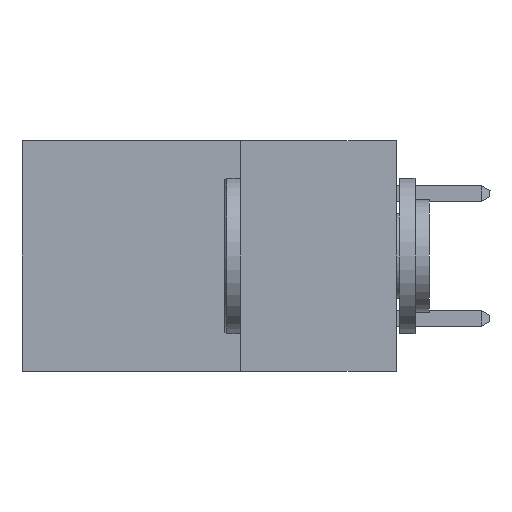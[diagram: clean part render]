
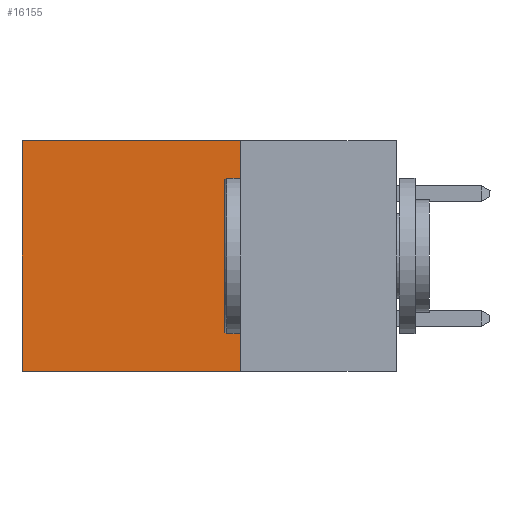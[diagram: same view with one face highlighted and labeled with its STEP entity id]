
A CAD part, left-side view. The second image highlights one B-rep face of the part: STEP entity #16155.
In plain terms, the highlighted planar face has unit normal (-1, 0, 0).
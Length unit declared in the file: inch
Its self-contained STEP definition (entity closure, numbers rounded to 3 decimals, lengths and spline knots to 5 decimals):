
#15 = LINE ( 'NONE', #16534, #13486 ) ;
#3151 = ORIENTED_EDGE ( 'NONE', *, *, #14069, .T. ) ;
#3170 = VECTOR ( 'NONE', #11652, 39.37008 ) ;
#3316 = EDGE_CURVE ( 'NONE', #9972, #3493, #14128, .T. ) ;
#3342 = EDGE_CURVE ( 'NONE', #8411, #16577, #3589, .T. ) ;
#3493 = VERTEX_POINT ( 'NONE', #13466 ) ;
#3589 = LINE ( 'NONE', #11911, #3170 ) ;
#3911 = CARTESIAN_POINT ( 'NONE',  ( 0.298, 0.25, 0. ) ) ;
#5063 = LINE ( 'NONE', #16751, #15480 ) ;
#5919 = ORIENTED_EDGE ( 'NONE', *, *, #3316, .T. ) ;
#6344 = ORIENTED_EDGE ( 'NONE', *, *, #8109, .F. ) ;
#6583 = PLANE ( 'NONE',  #7246 ) ;
#6640 = DIRECTION ( 'NONE',  ( 0., 0., -1. ) ) ;
#7246 = AXIS2_PLACEMENT_3D ( 'NONE', #3911, #14449, #6640 ) ;
#7383 = CARTESIAN_POINT ( 'NONE',  ( 0.298, 0.6, 0. ) ) ;
#7765 = DIRECTION ( 'NONE',  ( 0., 1., 0. ) ) ;
#8109 = EDGE_CURVE ( 'NONE', #16577, #3493, #5063, .T. ) ;
#8411 = VERTEX_POINT ( 'NONE', #10928 ) ;
#8626 = CARTESIAN_POINT ( 'NONE',  ( 0.298, 0.25, -0.37 ) ) ;
#9972 = VERTEX_POINT ( 'NONE', #7383 ) ;
#10173 = DIRECTION ( 'NONE',  ( 0., 1., 0. ) ) ;
#10680 = VECTOR ( 'NONE', #16764, 39.37008 ) ;
#10928 = CARTESIAN_POINT ( 'NONE',  ( 0.298, 0.25, 0. ) ) ;
#11652 = DIRECTION ( 'NONE',  ( 0., 0., -1. ) ) ;
#11911 = CARTESIAN_POINT ( 'NONE',  ( 0.298, 0.25, 0. ) ) ;
#13466 = CARTESIAN_POINT ( 'NONE',  ( 0.298, 0.6, -0.37 ) ) ;
#13486 = VECTOR ( 'NONE', #10173, 39.37008 ) ;
#14069 = EDGE_CURVE ( 'NONE', #8411, #9972, #15, .T. ) ;
#14128 = LINE ( 'NONE', #16730, #10680 ) ;
#14449 = DIRECTION ( 'NONE',  ( 1., 0., 0. ) ) ;
#15006 = FACE_OUTER_BOUND ( 'NONE', #16203, .T. ) ;
#15480 = VECTOR ( 'NONE', #7765, 39.37008 ) ;
#16155 = ADVANCED_FACE ( 'NONE', ( #15006 ), #6583, .F. ) ;
#16203 = EDGE_LOOP ( 'NONE', ( #5919, #6344, #16611, #3151 ) ) ;
#16534 = CARTESIAN_POINT ( 'NONE',  ( 0.298, 0.25, 0. ) ) ;
#16577 = VERTEX_POINT ( 'NONE', #8626 ) ;
#16611 = ORIENTED_EDGE ( 'NONE', *, *, #3342, .F. ) ;
#16730 = CARTESIAN_POINT ( 'NONE',  ( 0.298, 0.6, 0. ) ) ;
#16751 = CARTESIAN_POINT ( 'NONE',  ( 0.298, 0.25, -0.37 ) ) ;
#16764 = DIRECTION ( 'NONE',  ( 0., 0., -1. ) ) ;
